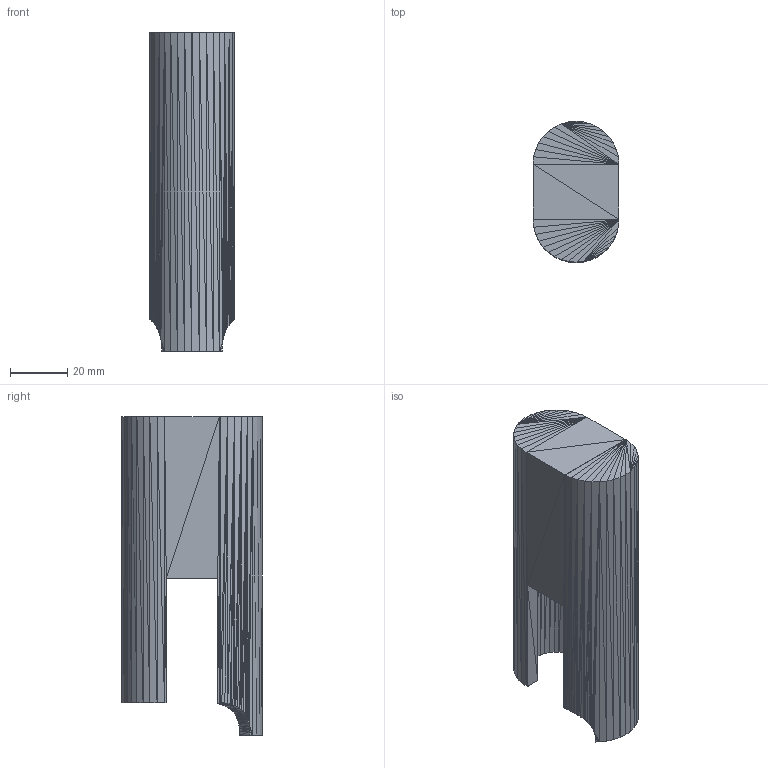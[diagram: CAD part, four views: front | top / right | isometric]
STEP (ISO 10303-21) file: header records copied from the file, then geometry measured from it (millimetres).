
FILE_DESCRIPTION (( 'STEP AP203' ), '1' );
FILE_NAME ('WeldingJig.STEP', '2020-06-09T22:12:01', ( '' ), ( '' ), 'SwSTEP 2.0', 'SolidWorks 2019', '' );
FILE_SCHEMA (( 'CONFIG_CONTROL_DESIGN' ));
Length unit declared in the file: millimetre
Products named in the file (1): WeldingJig
Bounding box: 30 x 49.2 x 111.3 mm (x, y, z)
Volume: 76392.9 mm3; surface area: 21675.7 mm2
Topology: 1 solids, 1 shells, 882 faces, 1333 edges, 453 vertices
Faces by surface type: plane 882
Entity records: 17378 total; most frequent: DIRECTION 3099, CARTESIAN_POINT 2669, ORIENTED_EDGE 2666, LINE 1333, EDGE_CURVE 1333, VECTOR 1333, AXIS2_PLACEMENT_3D 883, EDGE_LOOP 882
